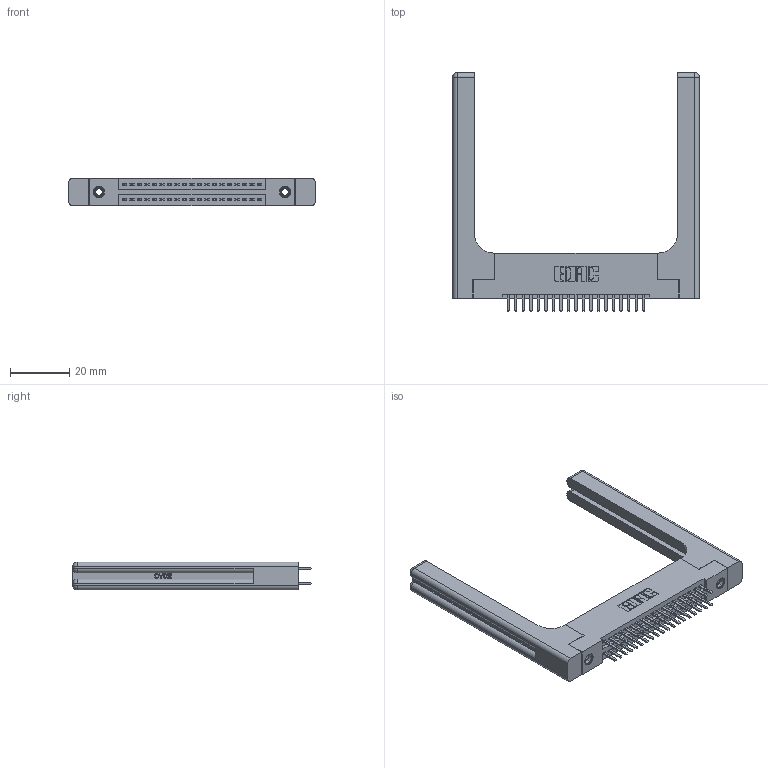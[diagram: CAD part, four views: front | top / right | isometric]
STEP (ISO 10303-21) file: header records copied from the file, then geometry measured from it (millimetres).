
FILE_DESCRIPTION (( 'STEP AP203' ), '1' );
FILE_NAME ('345-038-520-258.STEP', '2019-10-28T13:39:44', ( '' ), ( '' ), 'SwSTEP 2.0', 'SolidWorks 2016', '' );
FILE_SCHEMA (( 'CONFIG_CONTROL_DESIGN' ));
Length unit declared in the file: inch
Products named in the file (5): 345-250-001_345-250-001-102; 345-038-520-258; 345 Part_Flush Mounting Lugs - 0.156 Dia-TH; 345-292-001_345-293-120; 345-220-058_345-220-058
Assembly tree (43 placements, depth 2):
  345-038-520-258
    345 Part_Flush Mounting Lugs - 0.156 Dia-TH
    345-292-001_345-293-120  x38
    345-250-001_345-250-001-102  x2
    345-220-058_345-220-058  x2
Bounding box: 83.29 x 80.64 x 9.4 mm (x, y, z)
Volume: 16335.5 mm3; surface area: 16196.8 mm2
Topology: 43 solids, 43 shells, 2434 faces, 6973 edges, 4526 vertices
Faces by surface type: plane 1558, cylinder 816, bspline 36, cone 12, sphere 8, torus 4
Entity records: 23300 total; most frequent: CARTESIAN_POINT 4933, ORIENTED_EDGE 3652, DIRECTION 3298, EDGE_CURVE 1826, VECTOR 1522, LINE 1522, VERTEX_POINT 1206, AXIS2_PLACEMENT_3D 888
